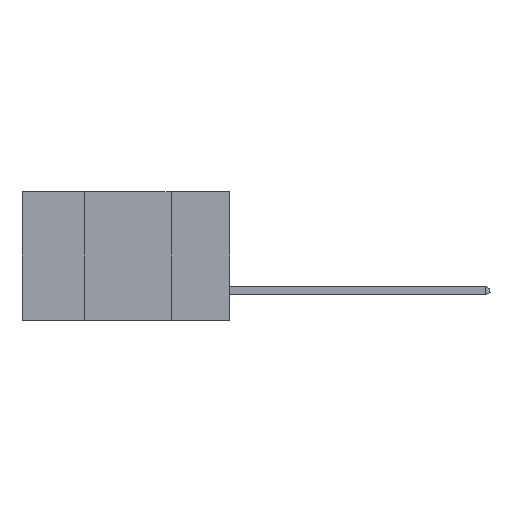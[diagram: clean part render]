
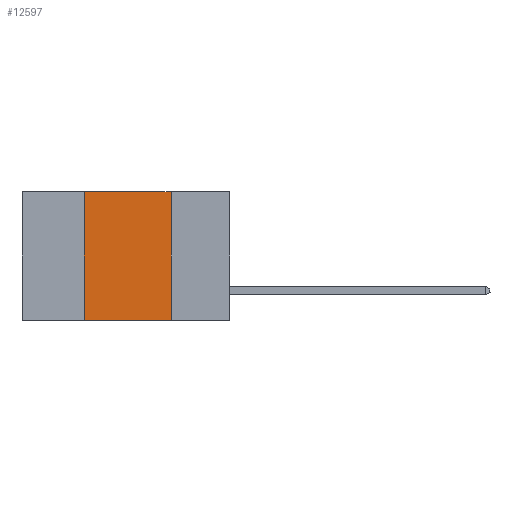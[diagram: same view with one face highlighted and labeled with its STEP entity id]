
A CAD part, left-side view. The second image highlights one B-rep face of the part: STEP entity #12597.
In plain terms, the highlighted planar face has unit normal (-1, 0, 0).
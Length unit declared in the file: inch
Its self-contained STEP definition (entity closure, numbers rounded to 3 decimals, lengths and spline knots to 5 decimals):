
#1543 = EDGE_CURVE ( 'NONE', #22915, #16046, #22469, .T. ) ;
#1824 = VERTEX_POINT ( 'NONE', #7910 ) ;
#2198 = EDGE_CURVE ( 'NONE', #22915, #8505, #29397, .T. ) ;
#3413 = ORIENTED_EDGE ( 'NONE', *, *, #26435, .F. ) ;
#3529 = CARTESIAN_POINT ( 'NONE',  ( 0., 0.42, 0. ) ) ;
#7910 = CARTESIAN_POINT ( 'NONE',  ( 0., 0.17, 0. ) ) ;
#8505 = VERTEX_POINT ( 'NONE', #3529 ) ;
#8749 = VECTOR ( 'NONE', #25147, 39.37008 ) ;
#8904 = ORIENTED_EDGE ( 'NONE', *, *, #1543, .T. ) ;
#9882 = VECTOR ( 'NONE', #29880, 39.37008 ) ;
#10098 = CARTESIAN_POINT ( 'NONE',  ( 0., 0.6, 0. ) ) ;
#10293 = VECTOR ( 'NONE', #21280, 39.37008 ) ;
#12326 = EDGE_CURVE ( 'NONE', #8505, #1824, #26884, .T. ) ;
#12597 = ADVANCED_FACE ( 'NONE', ( #23591 ), #23965, .F. ) ;
#12740 = VECTOR ( 'NONE', #26812, 39.37008 ) ;
#13149 = CARTESIAN_POINT ( 'NONE',  ( 0., 0.6, -0.37 ) ) ;
#15146 = DIRECTION ( 'NONE',  ( 0., 0., -1. ) ) ;
#15571 = CARTESIAN_POINT ( 'NONE',  ( 0., 0.42, -0.37 ) ) ;
#16046 = VERTEX_POINT ( 'NONE', #16749 ) ;
#16452 = LINE ( 'NONE', #21076, #10293 ) ;
#16749 = CARTESIAN_POINT ( 'NONE',  ( 0., 0.17, -0.37 ) ) ;
#21076 = CARTESIAN_POINT ( 'NONE',  ( 0., 0.17, 0. ) ) ;
#21280 = DIRECTION ( 'NONE',  ( 0., 0., -1. ) ) ;
#22469 = LINE ( 'NONE', #13149, #12740 ) ;
#22856 = AXIS2_PLACEMENT_3D ( 'NONE', #10098, #26281, #15146 ) ;
#22915 = VERTEX_POINT ( 'NONE', #15571 ) ;
#23591 = FACE_OUTER_BOUND ( 'NONE', #28549, .T. ) ;
#23965 = PLANE ( 'NONE',  #22856 ) ;
#25147 = DIRECTION ( 'NONE',  ( 0., 0., 1. ) ) ;
#26281 = DIRECTION ( 'NONE',  ( 1., 0., 0. ) ) ;
#26435 = EDGE_CURVE ( 'NONE', #1824, #16046, #16452, .T. ) ;
#26812 = DIRECTION ( 'NONE',  ( 0., -1., 0. ) ) ;
#26884 = LINE ( 'NONE', #27632, #9882 ) ;
#27183 = CARTESIAN_POINT ( 'NONE',  ( 0., 0.42, 0. ) ) ;
#27348 = ORIENTED_EDGE ( 'NONE', *, *, #2198, .F. ) ;
#27632 = CARTESIAN_POINT ( 'NONE',  ( 0., 0.6, 0. ) ) ;
#27813 = ORIENTED_EDGE ( 'NONE', *, *, #12326, .F. ) ;
#28549 = EDGE_LOOP ( 'NONE', ( #3413, #27813, #27348, #8904 ) ) ;
#29397 = LINE ( 'NONE', #27183, #8749 ) ;
#29880 = DIRECTION ( 'NONE',  ( 0., -1., 0. ) ) ;
